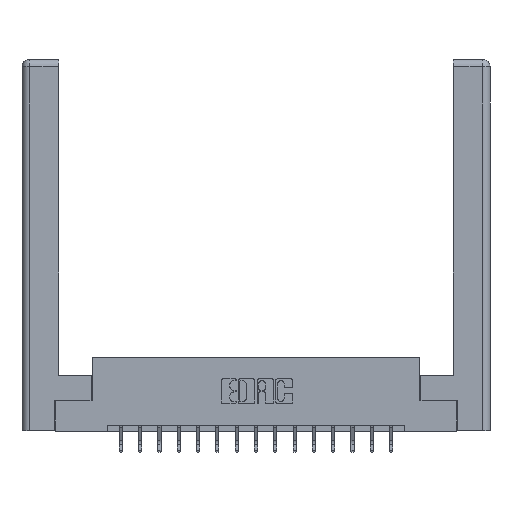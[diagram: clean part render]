
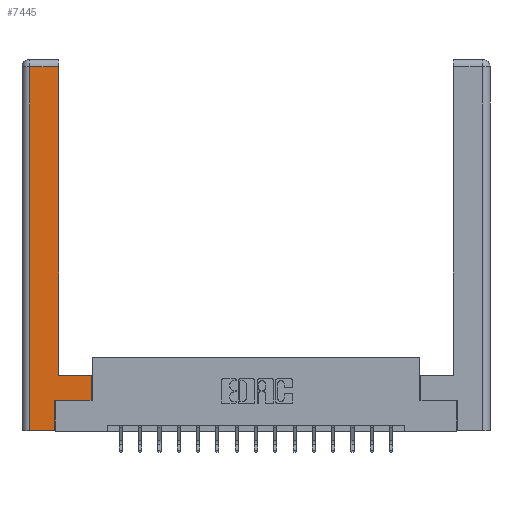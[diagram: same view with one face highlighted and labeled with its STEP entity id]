
A CAD part, top view. The second image highlights one B-rep face of the part: STEP entity #7445.
In plain terms, the highlighted planar face has unit normal (0, 0, 1).
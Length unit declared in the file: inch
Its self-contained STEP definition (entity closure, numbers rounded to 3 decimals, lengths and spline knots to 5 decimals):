
#24 = LINE ( 'NONE', #48, #1352 ) ;
#48 = CARTESIAN_POINT ( 'NONE',  ( 0.295, 0.45, 0. ) ) ;
#308 = EDGE_CURVE ( 'NONE', #8879, #11763, #8138, .T. ) ;
#1055 = EDGE_CURVE ( 'NONE', #3111, #3847, #17679, .T. ) ;
#1352 = VECTOR ( 'NONE', #6801, 39.37008 ) ;
#2266 = VERTEX_POINT ( 'NONE', #13616 ) ;
#2272 = DIRECTION ( 'NONE',  ( 0., 0., -1. ) ) ;
#2307 = DIRECTION ( 'NONE',  ( 1., 0., 0. ) ) ;
#2415 = LINE ( 'NONE', #2735, #16741 ) ;
#2520 = DIRECTION ( 'NONE',  ( 0., 1., 0. ) ) ;
#2735 = CARTESIAN_POINT ( 'NONE',  ( 0.265, 0., 0. ) ) ;
#3111 = VERTEX_POINT ( 'NONE', #3199 ) ;
#3199 = CARTESIAN_POINT ( 'NONE',  ( 0.295, 0.45, 0. ) ) ;
#3480 = DIRECTION ( 'NONE',  ( -1., 0., 0. ) ) ;
#3712 = VECTOR ( 'NONE', #3480, 39.37008 ) ;
#3847 = VERTEX_POINT ( 'NONE', #4258 ) ;
#4139 = FACE_OUTER_BOUND ( 'NONE', #13490, .T. ) ;
#4258 = CARTESIAN_POINT ( 'NONE',  ( 0.295, 2.94, 0. ) ) ;
#5135 = ORIENTED_EDGE ( 'NONE', *, *, #5345, .T. ) ;
#5345 = EDGE_CURVE ( 'NONE', #11763, #7005, #14828, .T. ) ;
#6801 = DIRECTION ( 'NONE',  ( -1., 0., 0. ) ) ;
#6936 = EDGE_CURVE ( 'NONE', #3847, #13383, #10640, .T. ) ;
#7005 = VERTEX_POINT ( 'NONE', #14786 ) ;
#7241 = DIRECTION ( 'NONE',  ( 0., -1., 0. ) ) ;
#7445 = ADVANCED_FACE ( 'NONE', ( #4139 ), #13426, .F. ) ;
#8138 = LINE ( 'NONE', #17290, #17464 ) ;
#8253 = ORIENTED_EDGE ( 'NONE', *, *, #15219, .T. ) ;
#8296 = CARTESIAN_POINT ( 'NONE',  ( 0.265, 0.245, 0. ) ) ;
#8581 = DIRECTION ( 'NONE',  ( 0., 1., 0. ) ) ;
#8753 = VECTOR ( 'NONE', #15158, 39.37008 ) ;
#8879 = VERTEX_POINT ( 'NONE', #8296 ) ;
#9105 = EDGE_CURVE ( 'NONE', #13710, #8879, #17677, .T. ) ;
#9462 = CARTESIAN_POINT ( 'NONE',  ( 0.565, 0.45, 0. ) ) ;
#9601 = DIRECTION ( 'NONE',  ( 1., 0., 0. ) ) ;
#10027 = ORIENTED_EDGE ( 'NONE', *, *, #6936, .T. ) ;
#10640 = LINE ( 'NONE', #15877, #3712 ) ;
#10847 = CARTESIAN_POINT ( 'NONE',  ( 0.295, 3., 0. ) ) ;
#11763 = VERTEX_POINT ( 'NONE', #17132 ) ;
#12558 = LINE ( 'NONE', #14144, #13440 ) ;
#12903 = ORIENTED_EDGE ( 'NONE', *, *, #308, .T. ) ;
#13260 = CARTESIAN_POINT ( 'NONE',  ( 0.265, 0., 0. ) ) ;
#13328 = CARTESIAN_POINT ( 'NONE',  ( 0.0615, 2.94, 0. ) ) ;
#13383 = VERTEX_POINT ( 'NONE', #13328 ) ;
#13426 = PLANE ( 'NONE',  #16163 ) ;
#13440 = VECTOR ( 'NONE', #7241, 39.37008 ) ;
#13486 = CARTESIAN_POINT ( 'NONE',  ( 0., 0., 0. ) ) ;
#13490 = EDGE_LOOP ( 'NONE', ( #15265, #10027, #14418, #16802, #14131, #12903, #5135, #8253 ) ) ;
#13616 = CARTESIAN_POINT ( 'NONE',  ( 0.0615, 0., 0. ) ) ;
#13710 = VERTEX_POINT ( 'NONE', #13260 ) ;
#14131 = ORIENTED_EDGE ( 'NONE', *, *, #9105, .T. ) ;
#14144 = CARTESIAN_POINT ( 'NONE',  ( 0.0615, 0., 0. ) ) ;
#14418 = ORIENTED_EDGE ( 'NONE', *, *, #16123, .T. ) ;
#14786 = CARTESIAN_POINT ( 'NONE',  ( 0.565, 0.45, 0. ) ) ;
#14828 = LINE ( 'NONE', #9462, #8753 ) ;
#15158 = DIRECTION ( 'NONE',  ( 0., 1., 0. ) ) ;
#15219 = EDGE_CURVE ( 'NONE', #7005, #3111, #24, .T. ) ;
#15265 = ORIENTED_EDGE ( 'NONE', *, *, #1055, .T. ) ;
#15273 = EDGE_CURVE ( 'NONE', #2266, #13710, #2415, .T. ) ;
#15877 = CARTESIAN_POINT ( 'NONE',  ( 0.0615, 2.94, 0. ) ) ;
#16123 = EDGE_CURVE ( 'NONE', #13383, #2266, #12558, .T. ) ;
#16163 = AXIS2_PLACEMENT_3D ( 'NONE', #13486, #2272, #17750 ) ;
#16741 = VECTOR ( 'NONE', #9601, 39.37008 ) ;
#16802 = ORIENTED_EDGE ( 'NONE', *, *, #15273, .T. ) ;
#16897 = CARTESIAN_POINT ( 'NONE',  ( 0.265, 0.245, 0. ) ) ;
#17006 = VECTOR ( 'NONE', #8581, 39.37008 ) ;
#17132 = CARTESIAN_POINT ( 'NONE',  ( 0.565, 0.245, 0. ) ) ;
#17230 = VECTOR ( 'NONE', #2520, 39.37008 ) ;
#17290 = CARTESIAN_POINT ( 'NONE',  ( 0.565, 0.245, 0. ) ) ;
#17464 = VECTOR ( 'NONE', #2307, 39.37008 ) ;
#17677 = LINE ( 'NONE', #16897, #17006 ) ;
#17679 = LINE ( 'NONE', #10847, #17230 ) ;
#17750 = DIRECTION ( 'NONE',  ( -1., 0., 0. ) ) ;
